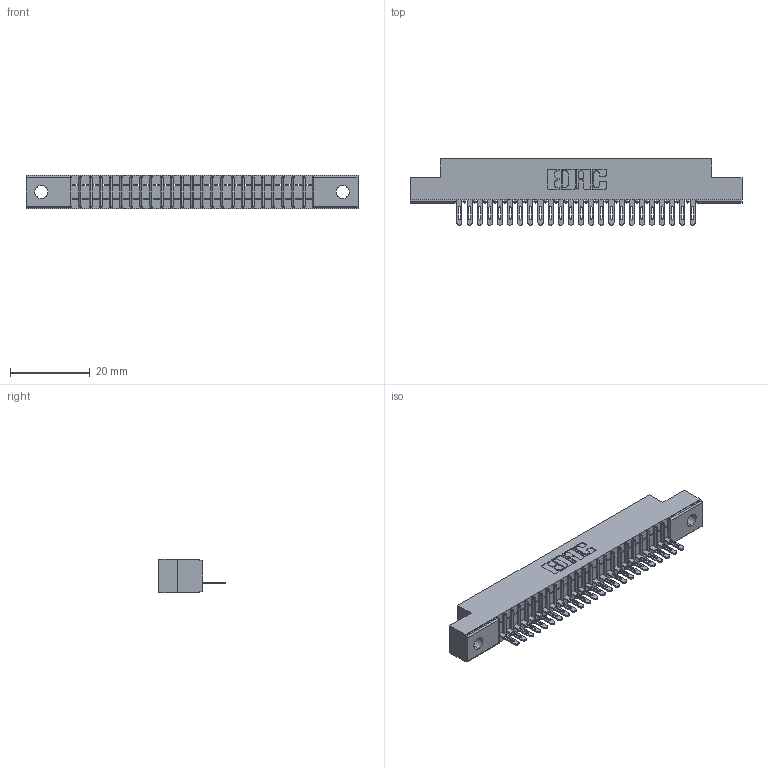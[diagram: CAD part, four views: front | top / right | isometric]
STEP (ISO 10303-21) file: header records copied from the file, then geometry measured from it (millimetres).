
FILE_DESCRIPTION (( 'STEP AP203' ), '1' );
FILE_NAME ('341-024-500-102.STEP', '2018-08-06T17:48:23', ( '' ), ( '' ), 'SwSTEP 2.0', 'SolidWorks 2016', '' );
FILE_SCHEMA (( 'CONFIG_CONTROL_DESIGN' ));
Length unit declared in the file: inch
Products named in the file (3): 341 Part_.128 (3.25) Dia Mounting Holes; 341-292-001_341-292-100; 341-024-500-102
Assembly tree (25 placements, depth 2):
  341-024-500-102
    341 Part_.128 (3.25) Dia Mounting Holes
    341-292-001_341-292-100  x24
Bounding box: 83.19 x 16.69 x 8.38 mm (x, y, z)
Volume: 4549.5 mm3; surface area: 8408.4 mm2
Topology: 25 solids, 25 shells, 2084 faces, 6004 edges, 3854 vertices
Faces by surface type: plane 1244, cylinder 744, sphere 50, torus 46
Entity records: 30685 total; most frequent: CARTESIAN_POINT 5204, ORIENTED_EDGE 5192, DIRECTION 5042, EDGE_CURVE 2596, LINE 2074, VECTOR 2074, VERTEX_POINT 1646, AXIS2_PLACEMENT_3D 1484
